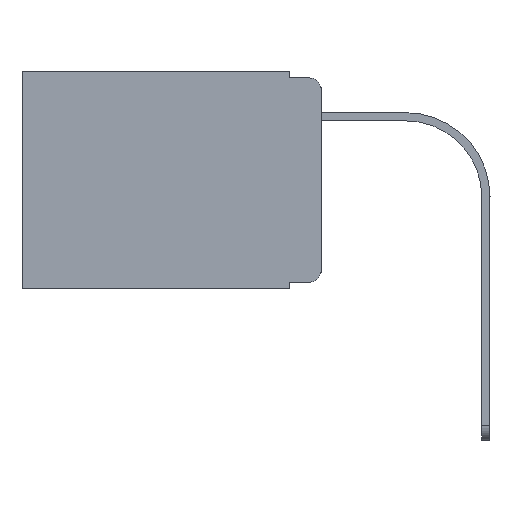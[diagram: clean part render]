
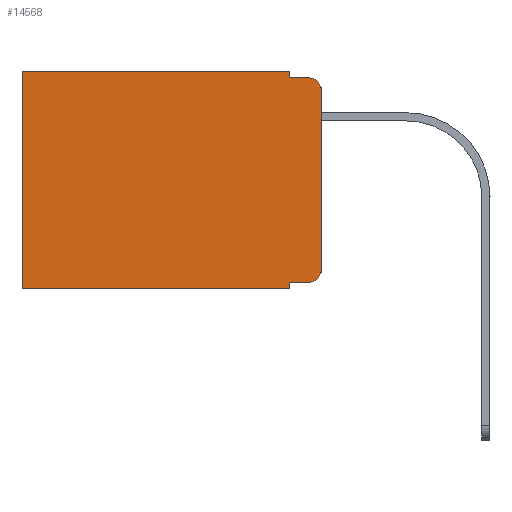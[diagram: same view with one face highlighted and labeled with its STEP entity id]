
A CAD part, left-side view. The second image highlights one B-rep face of the part: STEP entity #14568.
In plain terms, the highlighted planar face has unit normal (-1, 0, 0).
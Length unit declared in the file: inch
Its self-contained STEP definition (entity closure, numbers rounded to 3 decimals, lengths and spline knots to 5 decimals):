
#76 = LINE ( 'NONE', #8283, #2365 ) ;
#362 = EDGE_LOOP ( 'NONE', ( #17142, #13566, #15615, #16376, #3473, #8733, #11675, #857, #16289, #5584 ) ) ;
#857 = ORIENTED_EDGE ( 'NONE', *, *, #17006, .F. ) ;
#1492 = CARTESIAN_POINT ( 'NONE',  ( 0.298, 0.051, -0.01 ) ) ;
#1983 = VERTEX_POINT ( 'NONE', #16515 ) ;
#2365 = VECTOR ( 'NONE', #16343, 39.37008 ) ;
#2383 = VERTEX_POINT ( 'NONE', #13161 ) ;
#2673 = VECTOR ( 'NONE', #16567, 39.37008 ) ;
#2686 = VERTEX_POINT ( 'NONE', #12630 ) ;
#2870 = CARTESIAN_POINT ( 'NONE',  ( 0.298, 0.02, -0.333 ) ) ;
#3473 = ORIENTED_EDGE ( 'NONE', *, *, #6051, .T. ) ;
#3880 = VERTEX_POINT ( 'NONE', #9978 ) ;
#3968 = VECTOR ( 'NONE', #14503, 39.37008 ) ;
#4052 = FACE_OUTER_BOUND ( 'NONE', #362, .T. ) ;
#4095 = CARTESIAN_POINT ( 'NONE',  ( 0.298, 0., 0. ) ) ;
#4568 = LINE ( 'NONE', #1492, #3968 ) ;
#4835 = CARTESIAN_POINT ( 'NONE',  ( 0.298, 0.02, -0.313 ) ) ;
#5019 = CARTESIAN_POINT ( 'NONE',  ( 0.298, 0.051, 0. ) ) ;
#5038 = LINE ( 'NONE', #8220, #6657 ) ;
#5158 = VERTEX_POINT ( 'NONE', #8699 ) ;
#5472 = LINE ( 'NONE', #4095, #7966 ) ;
#5584 = ORIENTED_EDGE ( 'NONE', *, *, #13454, .T. ) ;
#6051 = EDGE_CURVE ( 'NONE', #15385, #6342, #5038, .T. ) ;
#6229 = EDGE_CURVE ( 'NONE', #10466, #3880, #4568, .T. ) ;
#6342 = VERTEX_POINT ( 'NONE', #13647 ) ;
#6657 = VECTOR ( 'NONE', #11534, 39.37008 ) ;
#7915 = AXIS2_PLACEMENT_3D ( 'NONE', #18195, #16272, #13360 ) ;
#7966 = VECTOR ( 'NONE', #20353, 39.37008 ) ;
#8182 = CARTESIAN_POINT ( 'NONE',  ( 0.298, 0.051, -0.01 ) ) ;
#8220 = CARTESIAN_POINT ( 'NONE',  ( 0.298, 0., 0. ) ) ;
#8283 = CARTESIAN_POINT ( 'NONE',  ( 0.298, 0., -0.343 ) ) ;
#8431 = DIRECTION ( 'NONE',  ( 0., 0., -1. ) ) ;
#8699 = CARTESIAN_POINT ( 'NONE',  ( 0.298, 0.051, -0.333 ) ) ;
#8733 = ORIENTED_EDGE ( 'NONE', *, *, #19777, .T. ) ;
#9357 = VERTEX_POINT ( 'NONE', #2870 ) ;
#9978 = CARTESIAN_POINT ( 'NONE',  ( 0.298, 0.02, -0.01 ) ) ;
#10321 = PLANE ( 'NONE',  #15485 ) ;
#10354 = EDGE_CURVE ( 'NONE', #1983, #18159, #76, .T. ) ;
#10466 = VERTEX_POINT ( 'NONE', #8182 ) ;
#10631 = AXIS2_PLACEMENT_3D ( 'NONE', #4835, #17465, #17778 ) ;
#10714 = CARTESIAN_POINT ( 'NONE',  ( 0.298, 0.473, -0.343 ) ) ;
#11534 = DIRECTION ( 'NONE',  ( 0., 1., 0. ) ) ;
#11675 = ORIENTED_EDGE ( 'NONE', *, *, #10354, .F. ) ;
#12145 = CARTESIAN_POINT ( 'NONE',  ( 0.298, 0., 0. ) ) ;
#12380 = EDGE_CURVE ( 'NONE', #2686, #3880, #12718, .T. ) ;
#12630 = CARTESIAN_POINT ( 'NONE',  ( 0.298, 0., -0.03 ) ) ;
#12718 = CIRCLE ( 'NONE', #7915, 0.02 ) ;
#13161 = CARTESIAN_POINT ( 'NONE',  ( 0.298, 0., -0.313 ) ) ;
#13240 = LINE ( 'NONE', #5019, #2673 ) ;
#13360 = DIRECTION ( 'NONE',  ( 0., 0., -1. ) ) ;
#13454 = EDGE_CURVE ( 'NONE', #9357, #2383, #17818, .T. ) ;
#13566 = ORIENTED_EDGE ( 'NONE', *, *, #12380, .T. ) ;
#13647 = CARTESIAN_POINT ( 'NONE',  ( 0.298, 0.473, 0. ) ) ;
#13949 = VECTOR ( 'NONE', #14872, 39.37008 ) ;
#13965 = CARTESIAN_POINT ( 'NONE',  ( 0.298, 0.051, -0.333 ) ) ;
#14064 = DIRECTION ( 'NONE',  ( 0., -1., 0. ) ) ;
#14503 = DIRECTION ( 'NONE',  ( 0., -1., 0. ) ) ;
#14547 = LINE ( 'NONE', #21096, #13949 ) ;
#14568 = ADVANCED_FACE ( 'NONE', ( #4052 ), #10321, .F. ) ;
#14872 = DIRECTION ( 'NONE',  ( 0., 0., -1. ) ) ;
#14982 = VECTOR ( 'NONE', #8431, 39.37008 ) ;
#14996 = CARTESIAN_POINT ( 'NONE',  ( 0.298, 0.051, 0. ) ) ;
#15247 = VECTOR ( 'NONE', #14064, 39.37008 ) ;
#15385 = VERTEX_POINT ( 'NONE', #14996 ) ;
#15485 = AXIS2_PLACEMENT_3D ( 'NONE', #12145, #18685, #17083 ) ;
#15597 = EDGE_CURVE ( 'NONE', #2686, #2383, #5472, .T. ) ;
#15615 = ORIENTED_EDGE ( 'NONE', *, *, #6229, .F. ) ;
#16272 = DIRECTION ( 'NONE',  ( -1., 0., 0. ) ) ;
#16289 = ORIENTED_EDGE ( 'NONE', *, *, #16518, .T. ) ;
#16343 = DIRECTION ( 'NONE',  ( 0., 1., 0. ) ) ;
#16376 = ORIENTED_EDGE ( 'NONE', *, *, #19865, .F. ) ;
#16515 = CARTESIAN_POINT ( 'NONE',  ( 0.298, 0.051, -0.343 ) ) ;
#16518 = EDGE_CURVE ( 'NONE', #5158, #9357, #17493, .T. ) ;
#16567 = DIRECTION ( 'NONE',  ( 0., 0., -1. ) ) ;
#16805 = LINE ( 'NONE', #18620, #14982 ) ;
#17006 = EDGE_CURVE ( 'NONE', #5158, #1983, #13240, .T. ) ;
#17083 = DIRECTION ( 'NONE',  ( 0., 0., -1. ) ) ;
#17142 = ORIENTED_EDGE ( 'NONE', *, *, #15597, .F. ) ;
#17465 = DIRECTION ( 'NONE',  ( -1., 0., 0. ) ) ;
#17493 = LINE ( 'NONE', #13965, #15247 ) ;
#17778 = DIRECTION ( 'NONE',  ( 0., 0., -1. ) ) ;
#17818 = CIRCLE ( 'NONE', #10631, 0.02 ) ;
#18159 = VERTEX_POINT ( 'NONE', #10714 ) ;
#18195 = CARTESIAN_POINT ( 'NONE',  ( 0.298, 0.02, -0.03 ) ) ;
#18620 = CARTESIAN_POINT ( 'NONE',  ( 0.298, 0.051, 0. ) ) ;
#18685 = DIRECTION ( 'NONE',  ( 1., 0., 0. ) ) ;
#19777 = EDGE_CURVE ( 'NONE', #6342, #18159, #14547, .T. ) ;
#19865 = EDGE_CURVE ( 'NONE', #15385, #10466, #16805, .T. ) ;
#20353 = DIRECTION ( 'NONE',  ( 0., 0., -1. ) ) ;
#21096 = CARTESIAN_POINT ( 'NONE',  ( 0.298, 0.473, 0. ) ) ;
